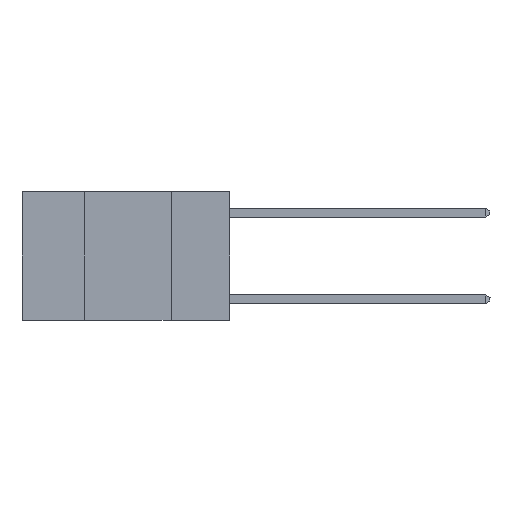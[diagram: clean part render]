
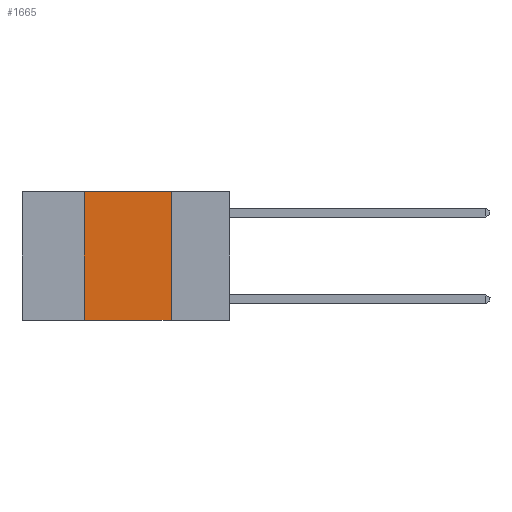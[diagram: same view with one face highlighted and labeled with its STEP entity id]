
A CAD part, left-side view. The second image highlights one B-rep face of the part: STEP entity #1665.
In plain terms, the highlighted planar face has unit normal (-1, 0, 0).
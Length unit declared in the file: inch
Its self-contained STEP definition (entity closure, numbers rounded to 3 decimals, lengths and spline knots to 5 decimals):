
#478 = ORIENTED_EDGE ( 'NONE', *, *, #14666, .T. ) ;
#1665 = ADVANCED_FACE ( 'NONE', ( #4766 ), #8280, .F. ) ;
#2143 = LINE ( 'NONE', #4504, #15612 ) ;
#2682 = DIRECTION ( 'NONE',  ( 0., 0., -1. ) ) ;
#2839 = CARTESIAN_POINT ( 'NONE',  ( 0., 0.17, -0.37 ) ) ;
#4293 = ORIENTED_EDGE ( 'NONE', *, *, #14670, .F. ) ;
#4504 = CARTESIAN_POINT ( 'NONE',  ( 0., 0.6, -0.37 ) ) ;
#4641 = CARTESIAN_POINT ( 'NONE',  ( 0., 0.6, 0. ) ) ;
#4766 = FACE_OUTER_BOUND ( 'NONE', #16488, .T. ) ;
#5983 = VECTOR ( 'NONE', #2682, 39.37008 ) ;
#6315 = VERTEX_POINT ( 'NONE', #15810 ) ;
#6520 = DIRECTION ( 'NONE',  ( 1., 0., 0. ) ) ;
#6740 = AXIS2_PLACEMENT_3D ( 'NONE', #4641, #6520, #19152 ) ;
#7341 = CARTESIAN_POINT ( 'NONE',  ( 0., 0.17, 0. ) ) ;
#8280 = PLANE ( 'NONE',  #6740 ) ;
#8535 = VERTEX_POINT ( 'NONE', #2839 ) ;
#9801 = CARTESIAN_POINT ( 'NONE',  ( 0., 0.42, -0.37 ) ) ;
#10000 = DIRECTION ( 'NONE',  ( 0., 0., 1. ) ) ;
#10879 = LINE ( 'NONE', #17163, #14537 ) ;
#11872 = CARTESIAN_POINT ( 'NONE',  ( 0., 0.17, 0. ) ) ;
#13992 = ORIENTED_EDGE ( 'NONE', *, *, #23215, .F. ) ;
#14537 = VECTOR ( 'NONE', #10000, 39.37008 ) ;
#14545 = ORIENTED_EDGE ( 'NONE', *, *, #22880, .F. ) ;
#14666 = EDGE_CURVE ( 'NONE', #16495, #8535, #2143, .T. ) ;
#14670 = EDGE_CURVE ( 'NONE', #16228, #8535, #20971, .T. ) ;
#15612 = VECTOR ( 'NONE', #22624, 39.37008 ) ;
#15810 = CARTESIAN_POINT ( 'NONE',  ( 0., 0.42, 0. ) ) ;
#16228 = VERTEX_POINT ( 'NONE', #7341 ) ;
#16277 = DIRECTION ( 'NONE',  ( 0., -1., 0. ) ) ;
#16488 = EDGE_LOOP ( 'NONE', ( #4293, #13992, #14545, #478 ) ) ;
#16495 = VERTEX_POINT ( 'NONE', #9801 ) ;
#16776 = LINE ( 'NONE', #21632, #21552 ) ;
#17163 = CARTESIAN_POINT ( 'NONE',  ( 0., 0.42, 0. ) ) ;
#19152 = DIRECTION ( 'NONE',  ( 0., 0., -1. ) ) ;
#20971 = LINE ( 'NONE', #11872, #5983 ) ;
#21552 = VECTOR ( 'NONE', #16277, 39.37008 ) ;
#21632 = CARTESIAN_POINT ( 'NONE',  ( 0., 0.6, 0. ) ) ;
#22624 = DIRECTION ( 'NONE',  ( 0., -1., 0. ) ) ;
#22880 = EDGE_CURVE ( 'NONE', #16495, #6315, #10879, .T. ) ;
#23215 = EDGE_CURVE ( 'NONE', #6315, #16228, #16776, .T. ) ;
